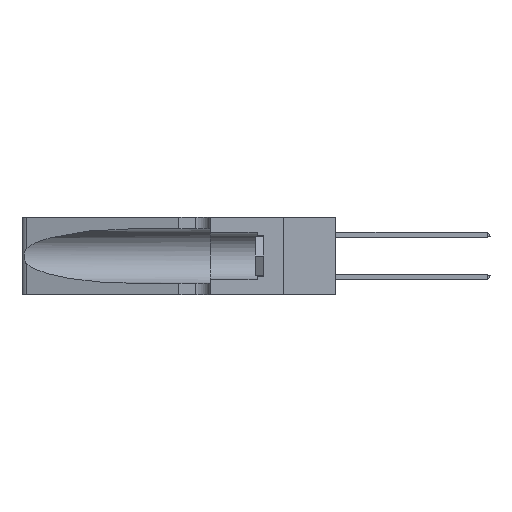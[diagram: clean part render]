
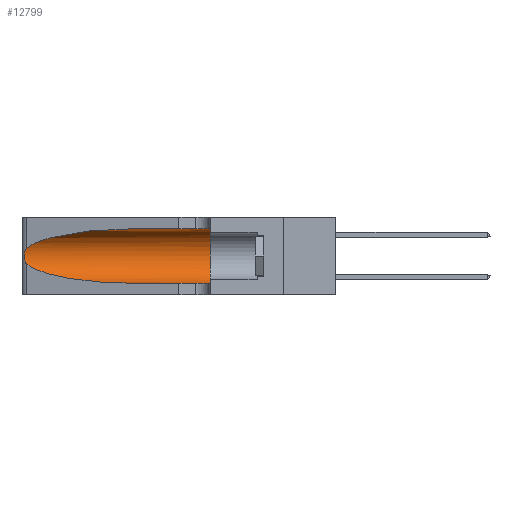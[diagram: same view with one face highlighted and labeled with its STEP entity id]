
A CAD part, left-side view. The second image highlights one B-rep face of the part: STEP entity #12799.
In plain terms, the highlighted cylindrical face has radius 3.308 mm (diameter 6.617 mm), a partial arc.
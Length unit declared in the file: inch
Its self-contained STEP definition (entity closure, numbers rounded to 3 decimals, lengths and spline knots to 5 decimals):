
#1653 = EDGE_CURVE ( 'NONE', #27469, #20000, #31750, .T. ) ;
#1750 = B_SPLINE_CURVE_WITH_KNOTS ( 'NONE', 3,
 ( #5177, #2426, #29553, #13336, #32184, #16105, #34836, #18838, #2540, #21546, #5289, #24260, #8004, #26973 ),
 .UNSPECIFIED., .F., .F.,
 ( 4, 2, 2, 2, 2, 2, 4 ),
 ( 0., 0.00027, 0.00053, 0.00107, 0.0016, 0.00187, 0.00214 ),
 .UNSPECIFIED. ) ;
#2426 = CARTESIAN_POINT ( 'NONE',  ( 0.25555, 1.22994, 0.2215 ) ) ;
#2540 = CARTESIAN_POINT ( 'NONE',  ( 0.26017, 1.23833, 0.17102 ) ) ;
#2845 = CARTESIAN_POINT ( 'NONE',  ( 0.1305, 1.61858, 0.31525 ) ) ;
#2915 = EDGE_CURVE ( 'NONE', #20000, #21799, #22455, .T. ) ;
#2986 = VECTOR ( 'NONE', #25749, 39.37008 ) ;
#3168 = DIRECTION ( 'NONE',  ( 0., -1., 0. ) ) ;
#4404 =( BOUNDED_CURVE ( )  B_SPLINE_CURVE ( 3, ( #11296, #8563, #19427, #30216 ),
 .UNSPECIFIED., .F., .T. ) 
 B_SPLINE_CURVE_WITH_KNOTS ( ( 4, 4 ),
 ( 3.44316, 4.71239 ),
 .UNSPECIFIED. ) 
 CURVE ( )  GEOMETRIC_REPRESENTATION_ITEM ( )  RATIONAL_B_SPLINE_CURVE ( ( 1., 0.87, 0.87, 1. ) ) 
 REPRESENTATION_ITEM ( '' )  );
#5177 = CARTESIAN_POINT ( 'NONE',  ( 0.25487, 1.22718, 0.22369 ) ) ;
#5184 = CARTESIAN_POINT ( 'NONE',  ( 0.18966, 0.96281, 0.31525 ) ) ;
#5289 = CARTESIAN_POINT ( 'NONE',  ( 0.25789, 1.23486, 0.15765 ) ) ;
#5427 = CARTESIAN_POINT ( 'NONE',  ( 0.1305, 0.35, 0.185 ) ) ;
#8004 = CARTESIAN_POINT ( 'NONE',  ( 0.25555, 1.22993, 0.14849 ) ) ;
#8020 = FACE_OUTER_BOUND ( 'NONE', #27605, .T. ) ;
#8142 = DIRECTION ( 'NONE',  ( 0., 0., 1. ) ) ;
#8320 = ORIENTED_EDGE ( 'NONE', *, *, #8545, .T. ) ;
#8508 = DIRECTION ( 'NONE',  ( 0., 0., -1. ) ) ;
#8545 = EDGE_CURVE ( 'NONE', #17636, #13989, #4404, .T. ) ;
#8563 = CARTESIAN_POINT ( 'NONE',  ( 0.2373, 1.15595, 0.08982 ) ) ;
#9669 = AXIS2_PLACEMENT_3D ( 'NONE', #27496, #13965, #8508 ) ;
#9880 = CARTESIAN_POINT ( 'NONE',  ( 0.25487, 1.22718, 0.14631 ) ) ;
#9982 = ORIENTED_EDGE ( 'NONE', *, *, #1653, .F. ) ;
#10011 = ORIENTED_EDGE ( 'NONE', *, *, #33550, .T. ) ;
#11296 = CARTESIAN_POINT ( 'NONE',  ( 0.25487, 1.22718, 0.14631 ) ) ;
#11763 =( BOUNDED_CURVE ( )  B_SPLINE_CURVE ( 3, ( #26865, #5184, #29557, #13341 ),
 .UNSPECIFIED., .F., .F. ) 
 B_SPLINE_CURVE_WITH_KNOTS ( ( 4, 4 ),
 ( 1.5708, 2.84003 ),
 .UNSPECIFIED. ) 
 CURVE ( )  GEOMETRIC_REPRESENTATION_ITEM ( )  RATIONAL_B_SPLINE_CURVE ( ( 1., 0.87, 0.87, 1. ) ) 
 REPRESENTATION_ITEM ( '' )  );
#12799 = ADVANCED_FACE ( 'NONE', ( #8020 ), #19948, .F. ) ;
#13336 = CARTESIAN_POINT ( 'NONE',  ( 0.25787, 1.23484, 0.2124 ) ) ;
#13341 = CARTESIAN_POINT ( 'NONE',  ( 0.25487, 1.22718, 0.22369 ) ) ;
#13965 = DIRECTION ( 'NONE',  ( 0., -1., 0. ) ) ;
#13989 = VERTEX_POINT ( 'NONE', #16576 ) ;
#15584 = ORIENTED_EDGE ( 'NONE', *, *, #28457, .T. ) ;
#16034 = VERTEX_POINT ( 'NONE', #16934 ) ;
#16105 = CARTESIAN_POINT ( 'NONE',  ( 0.26018, 1.23835, 0.19895 ) ) ;
#16576 = CARTESIAN_POINT ( 'NONE',  ( 0.1305, 0.72297, 0.05475 ) ) ;
#16934 = CARTESIAN_POINT ( 'NONE',  ( 0.25487, 1.22718, 0.22369 ) ) ;
#17636 = VERTEX_POINT ( 'NONE', #9880 ) ;
#18838 = CARTESIAN_POINT ( 'NONE',  ( 0.26075, 1.23896, 0.178 ) ) ;
#18962 = ORIENTED_EDGE ( 'NONE', *, *, #2915, .F. ) ;
#19427 = CARTESIAN_POINT ( 'NONE',  ( 0.18966, 0.96281, 0.05475 ) ) ;
#19497 = CARTESIAN_POINT ( 'NONE',  ( 0.1305, 0.72297, 0.31525 ) ) ;
#19948 = CYLINDRICAL_SURFACE ( 'NONE', #9669, 0.13025 ) ;
#20000 = VERTEX_POINT ( 'NONE', #30327 ) ;
#20699 = LINE ( 'NONE', #30153, #33229 ) ;
#21546 = CARTESIAN_POINT ( 'NONE',  ( 0.25856, 1.23593, 0.16098 ) ) ;
#21799 = VERTEX_POINT ( 'NONE', #31094 ) ;
#22455 = CIRCLE ( 'NONE', #23362, 0.13025 ) ;
#23200 = ORIENTED_EDGE ( 'NONE', *, *, #31348, .T. ) ;
#23362 = AXIS2_PLACEMENT_3D ( 'NONE', #5427, #24406, #8142 ) ;
#24260 = CARTESIAN_POINT ( 'NONE',  ( 0.25639, 1.23186, 0.15144 ) ) ;
#24406 = DIRECTION ( 'NONE',  ( 0., 1., 0. ) ) ;
#25749 = DIRECTION ( 'NONE',  ( 0., -1., 0. ) ) ;
#26865 = CARTESIAN_POINT ( 'NONE',  ( 0.1305, 0.72297, 0.31525 ) ) ;
#26973 = CARTESIAN_POINT ( 'NONE',  ( 0.25487, 1.22718, 0.14631 ) ) ;
#27469 = VERTEX_POINT ( 'NONE', #19497 ) ;
#27496 = CARTESIAN_POINT ( 'NONE',  ( 0.1305, 1.61858, 0.185 ) ) ;
#27605 = EDGE_LOOP ( 'NONE', ( #10011, #15584, #8320, #23200, #18962, #9982 ) ) ;
#28457 = EDGE_CURVE ( 'NONE', #16034, #17636, #1750, .T. ) ;
#29553 = CARTESIAN_POINT ( 'NONE',  ( 0.25639, 1.23184, 0.21858 ) ) ;
#29557 = CARTESIAN_POINT ( 'NONE',  ( 0.2373, 1.15595, 0.28018 ) ) ;
#30153 = CARTESIAN_POINT ( 'NONE',  ( 0.1305, 1.61858, 0.05475 ) ) ;
#30216 = CARTESIAN_POINT ( 'NONE',  ( 0.1305, 0.72297, 0.05475 ) ) ;
#30327 = CARTESIAN_POINT ( 'NONE',  ( 0.1305, 0.35, 0.31525 ) ) ;
#31094 = CARTESIAN_POINT ( 'NONE',  ( 0.1305, 0.35, 0.05475 ) ) ;
#31348 = EDGE_CURVE ( 'NONE', #13989, #21799, #20699, .T. ) ;
#31750 = LINE ( 'NONE', #2845, #2986 ) ;
#32184 = CARTESIAN_POINT ( 'NONE',  ( 0.25854, 1.2359, 0.20912 ) ) ;
#33229 = VECTOR ( 'NONE', #3168, 39.37008 ) ;
#33550 = EDGE_CURVE ( 'NONE', #27469, #16034, #11763, .T. ) ;
#34836 = CARTESIAN_POINT ( 'NONE',  ( 0.26075, 1.23896, 0.19203 ) ) ;
